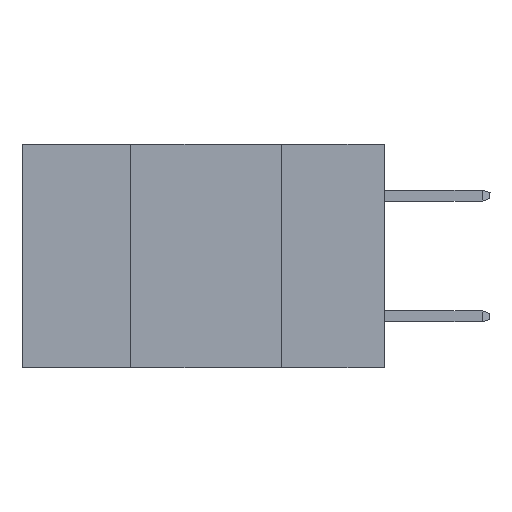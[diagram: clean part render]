
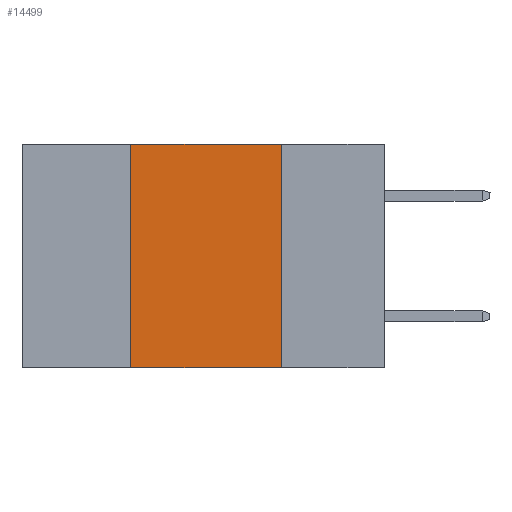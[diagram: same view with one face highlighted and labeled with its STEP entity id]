
A CAD part, left-side view. The second image highlights one B-rep face of the part: STEP entity #14499.
In plain terms, the highlighted planar face has unit normal (-1, 0, 0).
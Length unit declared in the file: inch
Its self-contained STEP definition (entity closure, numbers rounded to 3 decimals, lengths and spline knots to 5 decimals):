
#222 = LINE ( 'NONE', #27511, #7312 ) ;
#1725 = VECTOR ( 'NONE', #14927, 39.37008 ) ;
#2546 = ORIENTED_EDGE ( 'NONE', *, *, #14912, .F. ) ;
#3816 = VECTOR ( 'NONE', #7958, 39.37008 ) ;
#4530 = LINE ( 'NONE', #5679, #3816 ) ;
#4933 = LINE ( 'NONE', #5703, #1725 ) ;
#5673 = PLANE ( 'NONE',  #24078 ) ;
#5679 = CARTESIAN_POINT ( 'NONE',  ( 0., 0.17, 0. ) ) ;
#5703 = CARTESIAN_POINT ( 'NONE',  ( 0., 0.6, -0.37 ) ) ;
#5778 = CARTESIAN_POINT ( 'NONE',  ( 0., 0.6, 0. ) ) ;
#7312 = VECTOR ( 'NONE', #20445, 39.37008 ) ;
#7958 = DIRECTION ( 'NONE',  ( 0., 0., -1. ) ) ;
#7966 = CARTESIAN_POINT ( 'NONE',  ( 0., 0.42, -0.37 ) ) ;
#8142 = CARTESIAN_POINT ( 'NONE',  ( 0., 0.42, 0. ) ) ;
#9661 = EDGE_CURVE ( 'NONE', #29316, #18107, #222, .T. ) ;
#9700 = FACE_OUTER_BOUND ( 'NONE', #14489, .T. ) ;
#10327 = DIRECTION ( 'NONE',  ( 1., 0., 0. ) ) ;
#11473 = LINE ( 'NONE', #25827, #14384 ) ;
#12291 = ORIENTED_EDGE ( 'NONE', *, *, #9661, .F. ) ;
#13399 = VERTEX_POINT ( 'NONE', #22643 ) ;
#13643 = ORIENTED_EDGE ( 'NONE', *, *, #17279, .T. ) ;
#14384 = VECTOR ( 'NONE', #26030, 39.37008 ) ;
#14489 = EDGE_LOOP ( 'NONE', ( #15956, #2546, #12291, #13643 ) ) ;
#14499 = ADVANCED_FACE ( 'NONE', ( #9700 ), #5673, .F. ) ;
#14912 = EDGE_CURVE ( 'NONE', #18107, #13399, #11473, .T. ) ;
#14927 = DIRECTION ( 'NONE',  ( 0., -1., 0. ) ) ;
#15956 = ORIENTED_EDGE ( 'NONE', *, *, #18148, .F. ) ;
#17279 = EDGE_CURVE ( 'NONE', #29316, #20227, #4933, .T. ) ;
#18107 = VERTEX_POINT ( 'NONE', #8142 ) ;
#18148 = EDGE_CURVE ( 'NONE', #13399, #20227, #4530, .T. ) ;
#20227 = VERTEX_POINT ( 'NONE', #28161 ) ;
#20445 = DIRECTION ( 'NONE',  ( 0., 0., 1. ) ) ;
#22643 = CARTESIAN_POINT ( 'NONE',  ( 0., 0.17, 0. ) ) ;
#24078 = AXIS2_PLACEMENT_3D ( 'NONE', #5778, #10327, #26374 ) ;
#25827 = CARTESIAN_POINT ( 'NONE',  ( 0., 0.6, 0. ) ) ;
#26030 = DIRECTION ( 'NONE',  ( 0., -1., 0. ) ) ;
#26374 = DIRECTION ( 'NONE',  ( 0., 0., -1. ) ) ;
#27511 = CARTESIAN_POINT ( 'NONE',  ( 0., 0.42, 0. ) ) ;
#28161 = CARTESIAN_POINT ( 'NONE',  ( 0., 0.17, -0.37 ) ) ;
#29316 = VERTEX_POINT ( 'NONE', #7966 ) ;
